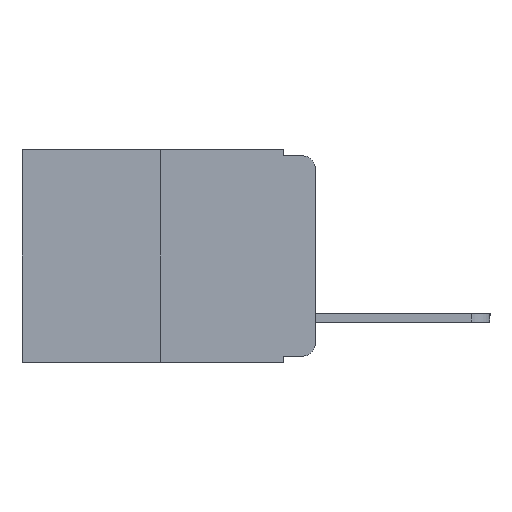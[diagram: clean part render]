
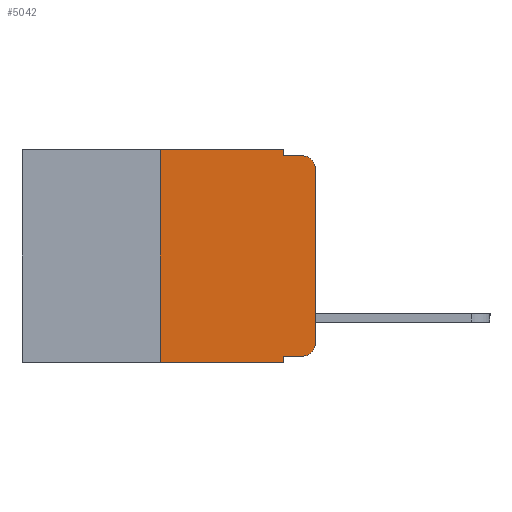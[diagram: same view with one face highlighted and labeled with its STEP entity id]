
A CAD part, left-side view. The second image highlights one B-rep face of the part: STEP entity #5042.
In plain terms, the highlighted planar face has unit normal (-1, 0, 0).
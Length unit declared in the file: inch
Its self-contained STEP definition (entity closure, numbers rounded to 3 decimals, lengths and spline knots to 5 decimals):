
#754 = ORIENTED_EDGE ( 'NONE', *, *, #20039, .T. ) ;
#878 = AXIS2_PLACEMENT_3D ( 'NONE', #17320, #12852, #6602 ) ;
#1041 = VERTEX_POINT ( 'NONE', #9420 ) ;
#1458 = CARTESIAN_POINT ( 'NONE',  ( 0., 0.051, 0. ) ) ;
#1762 = CARTESIAN_POINT ( 'NONE',  ( 0., 0.051, -0.333 ) ) ;
#2060 = DIRECTION ( 'NONE',  ( 0., -1., 0. ) ) ;
#2070 = CARTESIAN_POINT ( 'NONE',  ( 0., 0.25, 0. ) ) ;
#2310 = CARTESIAN_POINT ( 'NONE',  ( 0., 0., 0. ) ) ;
#2545 = DIRECTION ( 'NONE',  ( -1., 0., 0. ) ) ;
#2777 = CIRCLE ( 'NONE', #3643, 0.02 ) ;
#3062 = ORIENTED_EDGE ( 'NONE', *, *, #14956, .F. ) ;
#3142 = DIRECTION ( 'NONE',  ( 0., 0., -1. ) ) ;
#3193 = EDGE_LOOP ( 'NONE', ( #754, #12076, #6437, #3062, #19364, #10446, #11876, #14089, #18554, #3814 ) ) ;
#3643 = AXIS2_PLACEMENT_3D ( 'NONE', #12132, #2545, #13617 ) ;
#3814 = ORIENTED_EDGE ( 'NONE', *, *, #9839, .T. ) ;
#3953 = DIRECTION ( 'NONE',  ( 0., 0., 1. ) ) ;
#3954 = VECTOR ( 'NONE', #19074, 39.37008 ) ;
#4025 = CARTESIAN_POINT ( 'NONE',  ( 0., 0.051, 0. ) ) ;
#4201 = CARTESIAN_POINT ( 'NONE',  ( 0., 0.02, -0.01 ) ) ;
#4501 = VECTOR ( 'NONE', #11430, 39.37008 ) ;
#4772 = VERTEX_POINT ( 'NONE', #19339 ) ;
#5042 = ADVANCED_FACE ( 'NONE', ( #6882 ), #6412, .F. ) ;
#5889 = CIRCLE ( 'NONE', #12673, 0.02 ) ;
#6010 = DIRECTION ( 'NONE',  ( -1., 0., 0. ) ) ;
#6412 = PLANE ( 'NONE',  #878 ) ;
#6437 = ORIENTED_EDGE ( 'NONE', *, *, #17014, .F. ) ;
#6602 = DIRECTION ( 'NONE',  ( 0., 0., -1. ) ) ;
#6882 = FACE_OUTER_BOUND ( 'NONE', #3193, .T. ) ;
#6906 = LINE ( 'NONE', #2310, #10625 ) ;
#7960 = LINE ( 'NONE', #20007, #11664 ) ;
#8726 = LINE ( 'NONE', #13024, #3954 ) ;
#8800 = CARTESIAN_POINT ( 'NONE',  ( 0., 0.051, -0.343 ) ) ;
#8913 = VERTEX_POINT ( 'NONE', #4201 ) ;
#8945 = VERTEX_POINT ( 'NONE', #10793 ) ;
#9025 = EDGE_CURVE ( 'NONE', #17227, #17185, #11423, .T. ) ;
#9125 = LINE ( 'NONE', #19378, #13711 ) ;
#9420 = CARTESIAN_POINT ( 'NONE',  ( 0., 0.051, -0.01 ) ) ;
#9839 = EDGE_CURVE ( 'NONE', #8945, #16165, #2777, .T. ) ;
#9860 = VECTOR ( 'NONE', #2060, 39.37008 ) ;
#10446 = ORIENTED_EDGE ( 'NONE', *, *, #13941, .F. ) ;
#10625 = VECTOR ( 'NONE', #3953, 39.37008 ) ;
#10793 = CARTESIAN_POINT ( 'NONE',  ( 0., 0.02, -0.333 ) ) ;
#10910 = EDGE_CURVE ( 'NONE', #4772, #8945, #16952, .T. ) ;
#11401 = CARTESIAN_POINT ( 'NONE',  ( 0., 0., -0.03 ) ) ;
#11423 = LINE ( 'NONE', #20263, #19004 ) ;
#11430 = DIRECTION ( 'NONE',  ( 0., -1., 0. ) ) ;
#11664 = VECTOR ( 'NONE', #13973, 39.37008 ) ;
#11702 = CARTESIAN_POINT ( 'NONE',  ( 0., 0.473, 0. ) ) ;
#11876 = ORIENTED_EDGE ( 'NONE', *, *, #9025, .T. ) ;
#12076 = ORIENTED_EDGE ( 'NONE', *, *, #19048, .T. ) ;
#12132 = CARTESIAN_POINT ( 'NONE',  ( 0., 0.02, -0.313 ) ) ;
#12516 = VECTOR ( 'NONE', #3142, 39.37008 ) ;
#12616 = CARTESIAN_POINT ( 'NONE',  ( 0., 0., -0.313 ) ) ;
#12637 = VERTEX_POINT ( 'NONE', #2070 ) ;
#12673 = AXIS2_PLACEMENT_3D ( 'NONE', #15343, #6010, #16869 ) ;
#12852 = DIRECTION ( 'NONE',  ( 1., 0., 0. ) ) ;
#12922 = EDGE_CURVE ( 'NONE', #4772, #17185, #7960, .T. ) ;
#13024 = CARTESIAN_POINT ( 'NONE',  ( 0., 0.051, -0.01 ) ) ;
#13539 = CARTESIAN_POINT ( 'NONE',  ( 0., 0.25, -0.343 ) ) ;
#13617 = DIRECTION ( 'NONE',  ( 0., 0., -1. ) ) ;
#13711 = VECTOR ( 'NONE', #14867, 39.37008 ) ;
#13941 = EDGE_CURVE ( 'NONE', #17227, #12637, #9125, .T. ) ;
#13973 = DIRECTION ( 'NONE',  ( 0., 0., -1. ) ) ;
#14089 = ORIENTED_EDGE ( 'NONE', *, *, #12922, .F. ) ;
#14465 = EDGE_CURVE ( 'NONE', #12637, #20089, #18469, .T. ) ;
#14867 = DIRECTION ( 'NONE',  ( 0., 0., 1. ) ) ;
#14956 = EDGE_CURVE ( 'NONE', #20089, #1041, #17015, .T. ) ;
#15343 = CARTESIAN_POINT ( 'NONE',  ( 0., 0.02, -0.03 ) ) ;
#15844 = DIRECTION ( 'NONE',  ( 0., -1., 0. ) ) ;
#16165 = VERTEX_POINT ( 'NONE', #12616 ) ;
#16869 = DIRECTION ( 'NONE',  ( 0., 0., -1. ) ) ;
#16952 = LINE ( 'NONE', #1762, #4501 ) ;
#17014 = EDGE_CURVE ( 'NONE', #1041, #8913, #8726, .T. ) ;
#17015 = LINE ( 'NONE', #1458, #12516 ) ;
#17185 = VERTEX_POINT ( 'NONE', #8800 ) ;
#17227 = VERTEX_POINT ( 'NONE', #13539 ) ;
#17320 = CARTESIAN_POINT ( 'NONE',  ( 0., 0.473, 0. ) ) ;
#18469 = LINE ( 'NONE', #11702, #9860 ) ;
#18554 = ORIENTED_EDGE ( 'NONE', *, *, #10910, .T. ) ;
#18636 = VERTEX_POINT ( 'NONE', #11401 ) ;
#19004 = VECTOR ( 'NONE', #15844, 39.37008 ) ;
#19048 = EDGE_CURVE ( 'NONE', #18636, #8913, #5889, .T. ) ;
#19074 = DIRECTION ( 'NONE',  ( 0., -1., 0. ) ) ;
#19339 = CARTESIAN_POINT ( 'NONE',  ( 0., 0.051, -0.333 ) ) ;
#19364 = ORIENTED_EDGE ( 'NONE', *, *, #14465, .F. ) ;
#19378 = CARTESIAN_POINT ( 'NONE',  ( 0., 0.25, 0. ) ) ;
#20007 = CARTESIAN_POINT ( 'NONE',  ( 0., 0.051, 0. ) ) ;
#20039 = EDGE_CURVE ( 'NONE', #16165, #18636, #6906, .T. ) ;
#20089 = VERTEX_POINT ( 'NONE', #4025 ) ;
#20263 = CARTESIAN_POINT ( 'NONE',  ( 0., 0.473, -0.343 ) ) ;
